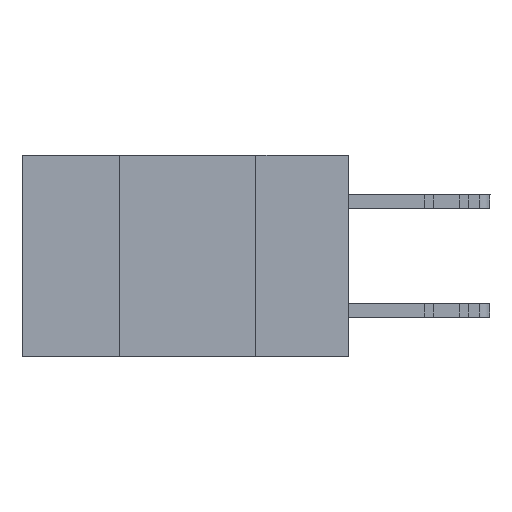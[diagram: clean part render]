
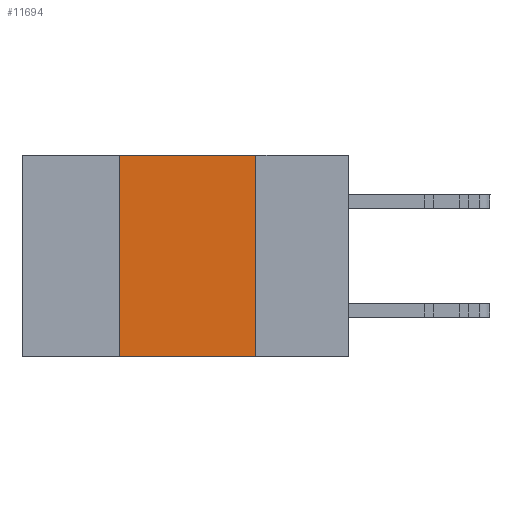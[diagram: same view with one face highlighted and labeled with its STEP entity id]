
A CAD part, left-side view. The second image highlights one B-rep face of the part: STEP entity #11694.
In plain terms, the highlighted planar face has unit normal (-1, 0, 0).
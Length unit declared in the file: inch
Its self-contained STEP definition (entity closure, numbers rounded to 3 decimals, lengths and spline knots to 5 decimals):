
#374 = EDGE_CURVE ( 'NONE', #25142, #30456, #14200, .T. ) ;
#1253 = LINE ( 'NONE', #20879, #24836 ) ;
#2968 = VERTEX_POINT ( 'NONE', #28267 ) ;
#3032 = EDGE_LOOP ( 'NONE', ( #26198, #28694, #19031, #9406 ) ) ;
#4478 = CARTESIAN_POINT ( 'NONE',  ( 0., 0.17, 0. ) ) ;
#5493 = FACE_OUTER_BOUND ( 'NONE', #3032, .T. ) ;
#5703 = EDGE_CURVE ( 'NONE', #30456, #15819, #1253, .T. ) ;
#6064 = EDGE_CURVE ( 'NONE', #2968, #15819, #20355, .T. ) ;
#6419 = CARTESIAN_POINT ( 'NONE',  ( 0., 0.6, -0.37 ) ) ;
#6471 = CARTESIAN_POINT ( 'NONE',  ( 0., 0.6, 0. ) ) ;
#7171 = CARTESIAN_POINT ( 'NONE',  ( 0., 0.42, 0. ) ) ;
#7407 = DIRECTION ( 'NONE',  ( 1., 0., 0. ) ) ;
#8767 = LINE ( 'NONE', #28078, #22022 ) ;
#8999 = DIRECTION ( 'NONE',  ( 0., -1., 0. ) ) ;
#9406 = ORIENTED_EDGE ( 'NONE', *, *, #6064, .T. ) ;
#9614 = CARTESIAN_POINT ( 'NONE',  ( 0., 0.6, 0. ) ) ;
#11694 = ADVANCED_FACE ( 'NONE', ( #5493 ), #29260, .F. ) ;
#12901 = VECTOR ( 'NONE', #8999, 39.37008 ) ;
#13756 = EDGE_CURVE ( 'NONE', #2968, #25142, #8767, .T. ) ;
#14200 = LINE ( 'NONE', #6471, #12901 ) ;
#15819 = VERTEX_POINT ( 'NONE', #29998 ) ;
#16604 = VECTOR ( 'NONE', #25716, 39.37008 ) ;
#19031 = ORIENTED_EDGE ( 'NONE', *, *, #13756, .F. ) ;
#20355 = LINE ( 'NONE', #6419, #16604 ) ;
#20879 = CARTESIAN_POINT ( 'NONE',  ( 0., 0.17, 0. ) ) ;
#22022 = VECTOR ( 'NONE', #30610, 39.37008 ) ;
#22633 = DIRECTION ( 'NONE',  ( 0., 0., -1. ) ) ;
#24836 = VECTOR ( 'NONE', #22633, 39.37008 ) ;
#25142 = VERTEX_POINT ( 'NONE', #7171 ) ;
#25522 = AXIS2_PLACEMENT_3D ( 'NONE', #9614, #7407, #29553 ) ;
#25716 = DIRECTION ( 'NONE',  ( 0., -1., 0. ) ) ;
#26198 = ORIENTED_EDGE ( 'NONE', *, *, #5703, .F. ) ;
#28078 = CARTESIAN_POINT ( 'NONE',  ( 0., 0.42, 0. ) ) ;
#28267 = CARTESIAN_POINT ( 'NONE',  ( 0., 0.42, -0.37 ) ) ;
#28694 = ORIENTED_EDGE ( 'NONE', *, *, #374, .F. ) ;
#29260 = PLANE ( 'NONE',  #25522 ) ;
#29553 = DIRECTION ( 'NONE',  ( 0., 0., -1. ) ) ;
#29998 = CARTESIAN_POINT ( 'NONE',  ( 0., 0.17, -0.37 ) ) ;
#30456 = VERTEX_POINT ( 'NONE', #4478 ) ;
#30610 = DIRECTION ( 'NONE',  ( 0., 0., 1. ) ) ;
